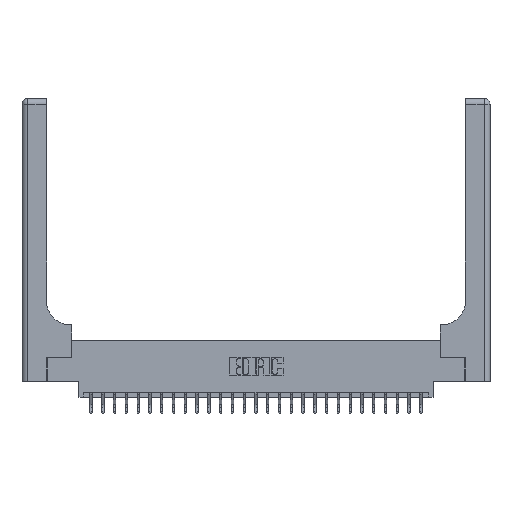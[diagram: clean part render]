
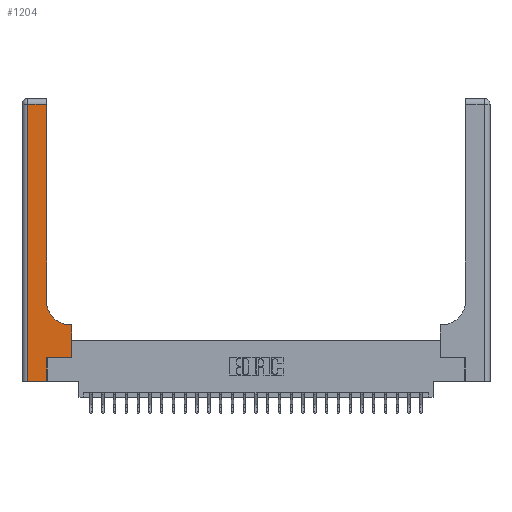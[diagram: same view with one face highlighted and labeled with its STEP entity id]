
A CAD part, top view. The second image highlights one B-rep face of the part: STEP entity #1204.
In plain terms, the highlighted planar face has unit normal (0, 0, 1).
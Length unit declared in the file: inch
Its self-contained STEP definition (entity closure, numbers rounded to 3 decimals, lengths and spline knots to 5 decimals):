
#84 = CIRCLE ( 'NONE', #17352, 0.25 ) ;
#614 = CARTESIAN_POINT ( 'NONE',  ( 0., 3., 0.37 ) ) ;
#635 = EDGE_CURVE ( 'NONE', #11611, #4222, #17435, .T. ) ;
#651 = LINE ( 'NONE', #12597, #22047 ) ;
#1103 = VECTOR ( 'NONE', #17872, 39.37008 ) ;
#1204 = ADVANCED_FACE ( 'NONE', ( #22639 ), #6295, .F. ) ;
#1920 = CARTESIAN_POINT ( 'NONE',  ( 0.06, 2.94, 0.37 ) ) ;
#2981 = CARTESIAN_POINT ( 'NONE',  ( 0.528, 0.6, 0.37 ) ) ;
#3007 = ORIENTED_EDGE ( 'NONE', *, *, #4629, .T. ) ;
#3261 = CARTESIAN_POINT ( 'NONE',  ( 0.26, 3., 0.37 ) ) ;
#3486 = EDGE_CURVE ( 'NONE', #11700, #6870, #23440, .T. ) ;
#3716 = DIRECTION ( 'NONE',  ( 1., 0., 0. ) ) ;
#3859 = LINE ( 'NONE', #20357, #17424 ) ;
#3966 = CARTESIAN_POINT ( 'NONE',  ( 0.265, 0., 0.37 ) ) ;
#4222 = VERTEX_POINT ( 'NONE', #1920 ) ;
#4629 = EDGE_CURVE ( 'NONE', #23450, #11611, #13940, .T. ) ;
#5508 = EDGE_CURVE ( 'NONE', #6698, #23450, #84, .T. ) ;
#6295 = PLANE ( 'NONE',  #16629 ) ;
#6527 = VECTOR ( 'NONE', #3716, 39.37008 ) ;
#6684 = DIRECTION ( 'NONE',  ( -1., 0., 0. ) ) ;
#6698 = VERTEX_POINT ( 'NONE', #11968 ) ;
#6745 = ORIENTED_EDGE ( 'NONE', *, *, #8989, .T. ) ;
#6838 = ORIENTED_EDGE ( 'NONE', *, *, #23365, .T. ) ;
#6870 = VERTEX_POINT ( 'NONE', #2981 ) ;
#7492 = CARTESIAN_POINT ( 'NONE',  ( 0.528, 0.25, 0.37 ) ) ;
#7533 = VECTOR ( 'NONE', #15257, 39.37008 ) ;
#7922 = DIRECTION ( 'NONE',  ( 0., -1., 0. ) ) ;
#8268 = CARTESIAN_POINT ( 'NONE',  ( 0.51, 0.85, 0.37 ) ) ;
#8793 = EDGE_LOOP ( 'NONE', ( #3007, #25664, #21444, #24610, #6838, #6745, #22923, #21685, #12056 ) ) ;
#8989 = EDGE_CURVE ( 'NONE', #15718, #11700, #15899, .T. ) ;
#10329 = LINE ( 'NONE', #3966, #10963 ) ;
#10364 = VERTEX_POINT ( 'NONE', #22534 ) ;
#10963 = VECTOR ( 'NONE', #12245, 39.37008 ) ;
#11074 = VECTOR ( 'NONE', #11087, 39.37008 ) ;
#11087 = DIRECTION ( 'NONE',  ( 1., 0., 0. ) ) ;
#11611 = VERTEX_POINT ( 'NONE', #20999 ) ;
#11700 = VERTEX_POINT ( 'NONE', #7492 ) ;
#11968 = CARTESIAN_POINT ( 'NONE',  ( 0.51, 0.6, 0.37 ) ) ;
#12056 = ORIENTED_EDGE ( 'NONE', *, *, #5508, .T. ) ;
#12245 = DIRECTION ( 'NONE',  ( 0., 1., 0. ) ) ;
#12597 = CARTESIAN_POINT ( 'NONE',  ( 0.26, 0.6, 0.37 ) ) ;
#13940 = LINE ( 'NONE', #3261, #1103 ) ;
#13965 = DIRECTION ( 'NONE',  ( 1., 0., 0. ) ) ;
#15050 = CARTESIAN_POINT ( 'NONE',  ( 0.26, 0.85, 0.37 ) ) ;
#15257 = DIRECTION ( 'NONE',  ( -1., 0., 0. ) ) ;
#15624 = CARTESIAN_POINT ( 'NONE',  ( 0.265, 0.25, 0.37 ) ) ;
#15718 = VERTEX_POINT ( 'NONE', #26442 ) ;
#15804 = CARTESIAN_POINT ( 'NONE',  ( 0., 2.94, 0.37 ) ) ;
#15899 = LINE ( 'NONE', #15624, #6527 ) ;
#16629 = AXIS2_PLACEMENT_3D ( 'NONE', #614, #18751, #6684 ) ;
#17024 = CARTESIAN_POINT ( 'NONE',  ( 0.06, 0., 0.37 ) ) ;
#17244 = DIRECTION ( 'NONE',  ( 0., 1., 0. ) ) ;
#17352 = AXIS2_PLACEMENT_3D ( 'NONE', #8268, #22191, #13965 ) ;
#17424 = VECTOR ( 'NONE', #7922, 39.37008 ) ;
#17435 = LINE ( 'NONE', #15804, #7533 ) ;
#17853 = LINE ( 'NONE', #22025, #11074 ) ;
#17872 = DIRECTION ( 'NONE',  ( 0., 1., 0. ) ) ;
#17919 = EDGE_CURVE ( 'NONE', #25714, #10364, #17853, .T. ) ;
#18573 = EDGE_CURVE ( 'NONE', #6870, #6698, #651, .T. ) ;
#18751 = DIRECTION ( 'NONE',  ( 0., 0., -1. ) ) ;
#20357 = CARTESIAN_POINT ( 'NONE',  ( 0.06, 3., 0.37 ) ) ;
#20665 = VECTOR ( 'NONE', #17244, 39.37008 ) ;
#20802 = DIRECTION ( 'NONE',  ( -1., 0., 0. ) ) ;
#20999 = CARTESIAN_POINT ( 'NONE',  ( 0.26, 2.94, 0.37 ) ) ;
#21444 = ORIENTED_EDGE ( 'NONE', *, *, #22010, .T. ) ;
#21685 = ORIENTED_EDGE ( 'NONE', *, *, #18573, .T. ) ;
#22010 = EDGE_CURVE ( 'NONE', #4222, #25714, #3859, .T. ) ;
#22025 = CARTESIAN_POINT ( 'NONE',  ( 0., 0., 0.37 ) ) ;
#22047 = VECTOR ( 'NONE', #20802, 39.37008 ) ;
#22191 = DIRECTION ( 'NONE',  ( 0., 0., -1. ) ) ;
#22534 = CARTESIAN_POINT ( 'NONE',  ( 0.265, 0., 0.37 ) ) ;
#22639 = FACE_OUTER_BOUND ( 'NONE', #8793, .T. ) ;
#22923 = ORIENTED_EDGE ( 'NONE', *, *, #3486, .T. ) ;
#23365 = EDGE_CURVE ( 'NONE', #10364, #15718, #10329, .T. ) ;
#23440 = LINE ( 'NONE', #25331, #20665 ) ;
#23450 = VERTEX_POINT ( 'NONE', #15050 ) ;
#24610 = ORIENTED_EDGE ( 'NONE', *, *, #17919, .T. ) ;
#25331 = CARTESIAN_POINT ( 'NONE',  ( 0.528, 0.25, 0.37 ) ) ;
#25664 = ORIENTED_EDGE ( 'NONE', *, *, #635, .T. ) ;
#25714 = VERTEX_POINT ( 'NONE', #17024 ) ;
#26442 = CARTESIAN_POINT ( 'NONE',  ( 0.265, 0.25, 0.37 ) ) ;
